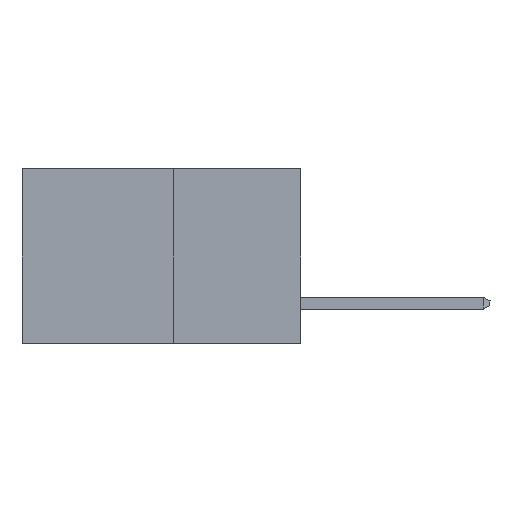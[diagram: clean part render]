
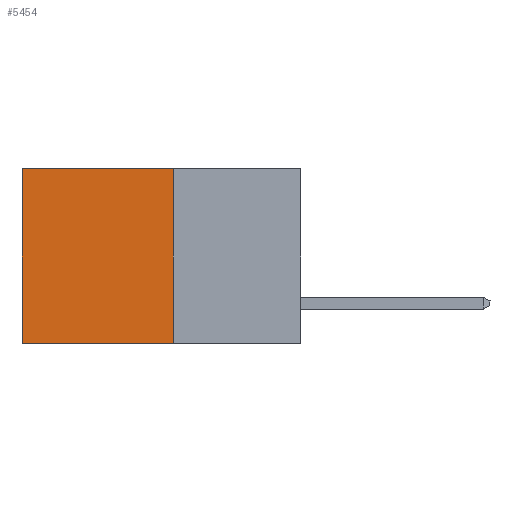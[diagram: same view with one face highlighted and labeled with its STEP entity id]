
A CAD part, left-side view. The second image highlights one B-rep face of the part: STEP entity #5454.
In plain terms, the highlighted planar face has unit normal (-1, 0, 0).
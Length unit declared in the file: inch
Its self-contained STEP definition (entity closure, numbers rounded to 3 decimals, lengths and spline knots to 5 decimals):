
#211 = VECTOR ( 'NONE', #2346, 39.37008 ) ;
#237 = ORIENTED_EDGE ( 'NONE', *, *, #3557, .T. ) ;
#422 = VECTOR ( 'NONE', #10011, 39.37008 ) ;
#688 = CARTESIAN_POINT ( 'NONE',  ( 0.277, 0.27, -0.37 ) ) ;
#1224 = EDGE_CURVE ( 'NONE', #1654, #4325, #7173, .T. ) ;
#1654 = VERTEX_POINT ( 'NONE', #8738 ) ;
#1847 = VERTEX_POINT ( 'NONE', #6281 ) ;
#2186 = EDGE_CURVE ( 'NONE', #5797, #1654, #5253, .T. ) ;
#2346 = DIRECTION ( 'NONE',  ( 0., 0., -1. ) ) ;
#2474 = CARTESIAN_POINT ( 'NONE',  ( 0.277, 0.27, -0.37 ) ) ;
#2611 = DIRECTION ( 'NONE',  ( 0., 1., 0. ) ) ;
#3557 = EDGE_CURVE ( 'NONE', #5797, #1847, #8741, .T. ) ;
#4085 = FACE_OUTER_BOUND ( 'NONE', #8456, .T. ) ;
#4261 = EDGE_CURVE ( 'NONE', #1847, #4325, #8124, .T. ) ;
#4325 = VERTEX_POINT ( 'NONE', #7297 ) ;
#4998 = CARTESIAN_POINT ( 'NONE',  ( 0.277, 0.27, 0. ) ) ;
#5031 = ORIENTED_EDGE ( 'NONE', *, *, #1224, .F. ) ;
#5253 = LINE ( 'NONE', #2474, #211 ) ;
#5273 = PLANE ( 'NONE',  #7977 ) ;
#5454 = ADVANCED_FACE ( 'NONE', ( #4085 ), #5273, .F. ) ;
#5797 = VERTEX_POINT ( 'NONE', #4998 ) ;
#6281 = CARTESIAN_POINT ( 'NONE',  ( 0.277, 0.59, 0. ) ) ;
#6356 = CARTESIAN_POINT ( 'NONE',  ( 0.277, 0.27, 0. ) ) ;
#6587 = ORIENTED_EDGE ( 'NONE', *, *, #4261, .T. ) ;
#6811 = DIRECTION ( 'NONE',  ( 0., 0., -1. ) ) ;
#7004 = VECTOR ( 'NONE', #2611, 39.37008 ) ;
#7173 = LINE ( 'NONE', #10051, #422 ) ;
#7297 = CARTESIAN_POINT ( 'NONE',  ( 0.277, 0.59, -0.37 ) ) ;
#7826 = DIRECTION ( 'NONE',  ( 1., 0., 0. ) ) ;
#7977 = AXIS2_PLACEMENT_3D ( 'NONE', #688, #7826, #6811 ) ;
#8124 = LINE ( 'NONE', #8141, #9830 ) ;
#8141 = CARTESIAN_POINT ( 'NONE',  ( 0.277, 0.59, -0.37 ) ) ;
#8456 = EDGE_LOOP ( 'NONE', ( #6587, #5031, #9315, #237 ) ) ;
#8700 = DIRECTION ( 'NONE',  ( 0., 0., -1. ) ) ;
#8738 = CARTESIAN_POINT ( 'NONE',  ( 0.277, 0.27, -0.37 ) ) ;
#8741 = LINE ( 'NONE', #6356, #7004 ) ;
#9315 = ORIENTED_EDGE ( 'NONE', *, *, #2186, .F. ) ;
#9830 = VECTOR ( 'NONE', #8700, 39.37008 ) ;
#10011 = DIRECTION ( 'NONE',  ( 0., 1., 0. ) ) ;
#10051 = CARTESIAN_POINT ( 'NONE',  ( 0.277, 0.27, -0.37 ) ) ;
